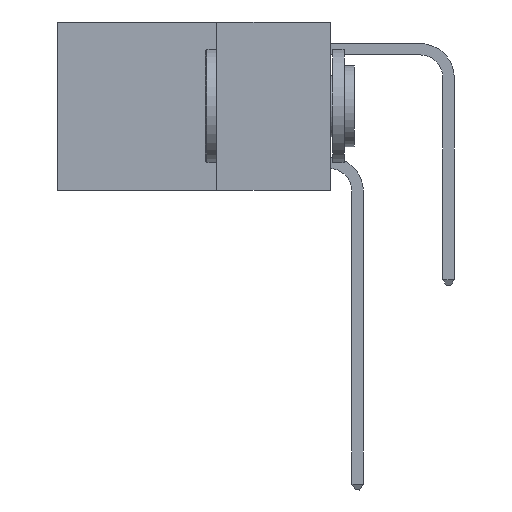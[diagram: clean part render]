
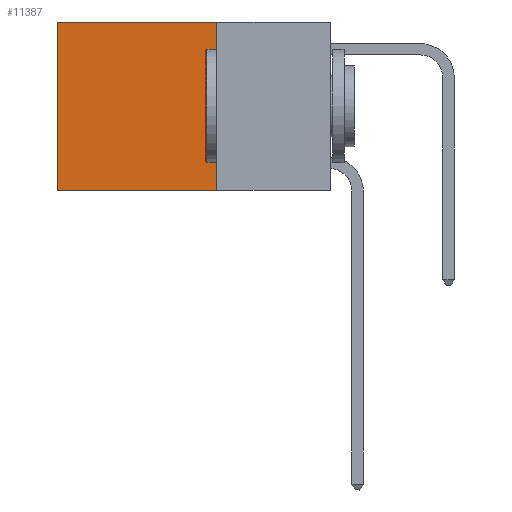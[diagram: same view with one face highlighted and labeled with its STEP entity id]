
A CAD part, left-side view. The second image highlights one B-rep face of the part: STEP entity #11387.
In plain terms, the highlighted planar face has unit normal (-1, 0, 0).
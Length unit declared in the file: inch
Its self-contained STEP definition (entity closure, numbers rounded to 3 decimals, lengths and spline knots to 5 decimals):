
#686 = LINE ( 'NONE', #9941, #8075 ) ;
#1307 = CARTESIAN_POINT ( 'NONE',  ( 0.2625, 0.25, -0.37 ) ) ;
#1509 = DIRECTION ( 'NONE',  ( 0., 1., 0. ) ) ;
#1555 = CARTESIAN_POINT ( 'NONE',  ( 0.2625, 0.25, 0. ) ) ;
#1602 = CARTESIAN_POINT ( 'NONE',  ( 0.2625, 0.6, -0.37 ) ) ;
#2701 = ORIENTED_EDGE ( 'NONE', *, *, #13531, .F. ) ;
#3095 = CARTESIAN_POINT ( 'NONE',  ( 0.2625, 0.25, 0. ) ) ;
#3105 = AXIS2_PLACEMENT_3D ( 'NONE', #1555, #3740, #11513 ) ;
#3154 = VECTOR ( 'NONE', #7864, 39.37008 ) ;
#3740 = DIRECTION ( 'NONE',  ( 1., 0., 0. ) ) ;
#3966 = ORIENTED_EDGE ( 'NONE', *, *, #11918, .T. ) ;
#4406 = LINE ( 'NONE', #11561, #11176 ) ;
#4843 = EDGE_LOOP ( 'NONE', ( #12340, #2701, #9686, #3966 ) ) ;
#5133 = FACE_OUTER_BOUND ( 'NONE', #4843, .T. ) ;
#6837 = LINE ( 'NONE', #3095, #10997 ) ;
#7706 = CARTESIAN_POINT ( 'NONE',  ( 0.2625, 0.25, 0. ) ) ;
#7740 = EDGE_CURVE ( 'NONE', #10470, #8318, #6837, .T. ) ;
#7864 = DIRECTION ( 'NONE',  ( 0., 1., 0. ) ) ;
#8075 = VECTOR ( 'NONE', #9899, 39.37008 ) ;
#8121 = CARTESIAN_POINT ( 'NONE',  ( 0.2625, 0.6, 0. ) ) ;
#8318 = VERTEX_POINT ( 'NONE', #11456 ) ;
#8843 = LINE ( 'NONE', #1307, #3154 ) ;
#9686 = ORIENTED_EDGE ( 'NONE', *, *, #7740, .F. ) ;
#9899 = DIRECTION ( 'NONE',  ( 0., 0., -1. ) ) ;
#9941 = CARTESIAN_POINT ( 'NONE',  ( 0.2625, 0.6, 0. ) ) ;
#10436 = EDGE_CURVE ( 'NONE', #14119, #11389, #686, .T. ) ;
#10441 = PLANE ( 'NONE',  #3105 ) ;
#10470 = VERTEX_POINT ( 'NONE', #7706 ) ;
#10703 = DIRECTION ( 'NONE',  ( 0., 0., -1. ) ) ;
#10997 = VECTOR ( 'NONE', #10703, 39.37008 ) ;
#11176 = VECTOR ( 'NONE', #1509, 39.37008 ) ;
#11387 = ADVANCED_FACE ( 'NONE', ( #5133 ), #10441, .F. ) ;
#11389 = VERTEX_POINT ( 'NONE', #1602 ) ;
#11456 = CARTESIAN_POINT ( 'NONE',  ( 0.2625, 0.25, -0.37 ) ) ;
#11513 = DIRECTION ( 'NONE',  ( 0., 0., -1. ) ) ;
#11561 = CARTESIAN_POINT ( 'NONE',  ( 0.2625, 0.25, 0. ) ) ;
#11918 = EDGE_CURVE ( 'NONE', #10470, #14119, #4406, .T. ) ;
#12340 = ORIENTED_EDGE ( 'NONE', *, *, #10436, .T. ) ;
#13531 = EDGE_CURVE ( 'NONE', #8318, #11389, #8843, .T. ) ;
#14119 = VERTEX_POINT ( 'NONE', #8121 ) ;
